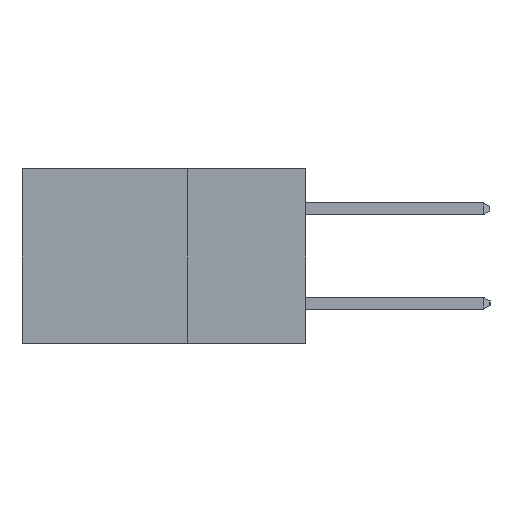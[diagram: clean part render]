
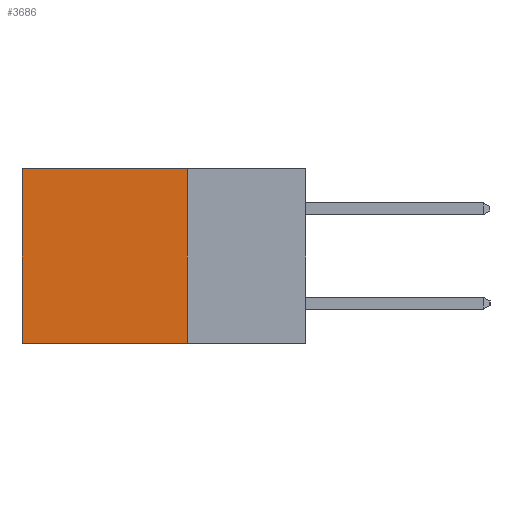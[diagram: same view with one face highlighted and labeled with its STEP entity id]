
A CAD part, left-side view. The second image highlights one B-rep face of the part: STEP entity #3686.
In plain terms, the highlighted planar face has unit normal (-1, 0, 0).
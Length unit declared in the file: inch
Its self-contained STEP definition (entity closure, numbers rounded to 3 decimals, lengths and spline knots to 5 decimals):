
#808 = ORIENTED_EDGE ( 'NONE', *, *, #6820, .T. ) ;
#908 = CARTESIAN_POINT ( 'NONE',  ( 0.2615, 0.6, -0.37 ) ) ;
#1127 = CARTESIAN_POINT ( 'NONE',  ( 0.2615, 0.25, -0.37 ) ) ;
#1301 = EDGE_CURVE ( 'NONE', #10262, #3792, #11351, .T. ) ;
#1953 = EDGE_LOOP ( 'NONE', ( #808, #7553, #9374, #9194 ) ) ;
#2182 = DIRECTION ( 'NONE',  ( 0., 0., -1. ) ) ;
#2440 = PLANE ( 'NONE',  #11774 ) ;
#3414 = DIRECTION ( 'NONE',  ( 0., 0., -1. ) ) ;
#3497 = CARTESIAN_POINT ( 'NONE',  ( 0.2615, 0.25, -0.37 ) ) ;
#3541 = LINE ( 'NONE', #8025, #12036 ) ;
#3686 = ADVANCED_FACE ( 'NONE', ( #9405 ), #2440, .F. ) ;
#3690 = CARTESIAN_POINT ( 'NONE',  ( 0.2615, 0.25, -0.37 ) ) ;
#3710 = CARTESIAN_POINT ( 'NONE',  ( 0.2615, 0.6, 0. ) ) ;
#3792 = VERTEX_POINT ( 'NONE', #908 ) ;
#4218 = DIRECTION ( 'NONE',  ( 0., 1., 0. ) ) ;
#4632 = VECTOR ( 'NONE', #8477, 39.37008 ) ;
#5884 = LINE ( 'NONE', #3497, #11632 ) ;
#5963 = EDGE_CURVE ( 'NONE', #10850, #11906, #3541, .T. ) ;
#6632 = DIRECTION ( 'NONE',  ( 0., 1., 0. ) ) ;
#6820 = EDGE_CURVE ( 'NONE', #11906, #3792, #8207, .T. ) ;
#7553 = ORIENTED_EDGE ( 'NONE', *, *, #1301, .F. ) ;
#8025 = CARTESIAN_POINT ( 'NONE',  ( 0.2615, 0.25, 0. ) ) ;
#8207 = LINE ( 'NONE', #8529, #4632 ) ;
#8477 = DIRECTION ( 'NONE',  ( 0., 0., -1. ) ) ;
#8529 = CARTESIAN_POINT ( 'NONE',  ( 0.2615, 0.6, -0.37 ) ) ;
#9101 = DIRECTION ( 'NONE',  ( 1., 0., 0. ) ) ;
#9119 = CARTESIAN_POINT ( 'NONE',  ( 0.2615, 0.25, -0.37 ) ) ;
#9194 = ORIENTED_EDGE ( 'NONE', *, *, #5963, .T. ) ;
#9374 = ORIENTED_EDGE ( 'NONE', *, *, #11925, .F. ) ;
#9405 = FACE_OUTER_BOUND ( 'NONE', #1953, .T. ) ;
#10262 = VERTEX_POINT ( 'NONE', #3690 ) ;
#10850 = VERTEX_POINT ( 'NONE', #11434 ) ;
#11028 = VECTOR ( 'NONE', #4218, 39.37008 ) ;
#11351 = LINE ( 'NONE', #1127, #11028 ) ;
#11434 = CARTESIAN_POINT ( 'NONE',  ( 0.2615, 0.25, 0. ) ) ;
#11632 = VECTOR ( 'NONE', #3414, 39.37008 ) ;
#11774 = AXIS2_PLACEMENT_3D ( 'NONE', #9119, #9101, #2182 ) ;
#11906 = VERTEX_POINT ( 'NONE', #3710 ) ;
#11925 = EDGE_CURVE ( 'NONE', #10850, #10262, #5884, .T. ) ;
#12036 = VECTOR ( 'NONE', #6632, 39.37008 ) ;
